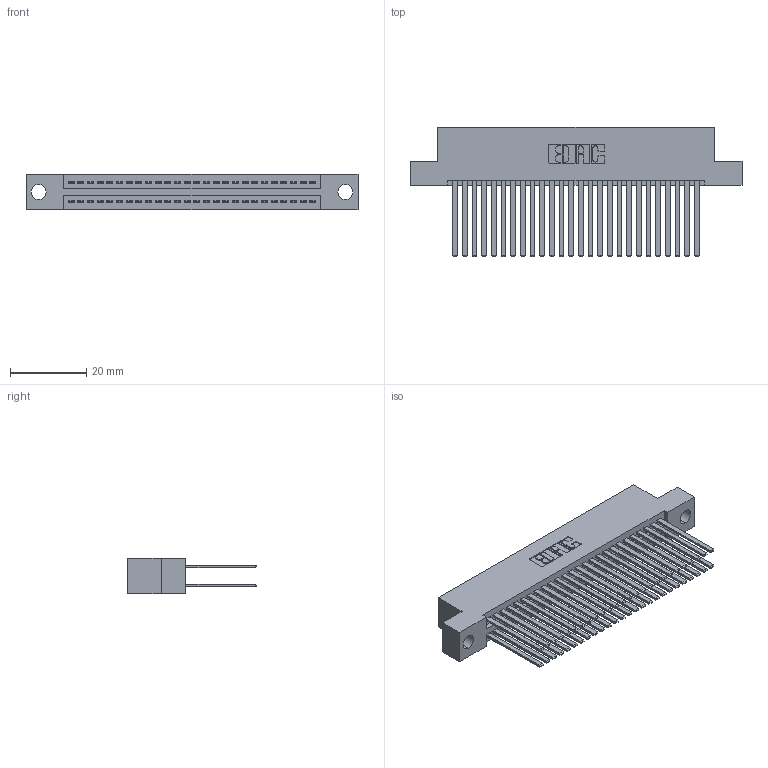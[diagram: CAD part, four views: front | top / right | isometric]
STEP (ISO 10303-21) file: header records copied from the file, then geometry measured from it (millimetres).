
FILE_DESCRIPTION (( 'STEP AP203' ), '1' );
FILE_NAME ('395-052-544-204.STEP', '2018-11-21T00:33:08', ( '' ), ( '' ), 'SwSTEP 2.0', 'SolidWorks 2016', '' );
FILE_SCHEMA (( 'CONFIG_CONTROL_DESIGN' ));
Length unit declared in the file: inch
Products named in the file (3): 395-052-544-204; 345 Part_Flush Mounting Lugs - 0.156 Dia-TH; 345-292-001_345-293-144
Assembly tree (53 placements, depth 2):
  395-052-544-204
    345 Part_Flush Mounting Lugs - 0.156 Dia-TH
    345-292-001_345-293-144  x52
Bounding box: 87.25 x 33.96 x 9.4 mm (x, y, z)
Volume: 8968 mm3; surface area: 14898 mm2
Topology: 53 solids, 53 shells, 2414 faces, 7153 edges, 4698 vertices
Faces by surface type: plane 1588, cylinder 826
Entity records: 22373 total; most frequent: CARTESIAN_POINT 3764, ORIENTED_EDGE 3698, DIRECTION 3337, EDGE_CURVE 1849, LINE 1617, VECTOR 1617, VERTEX_POINT 1230, AXIS2_PLACEMENT_3D 860
